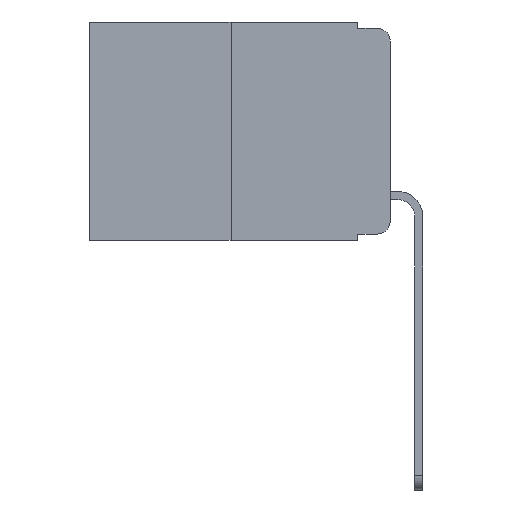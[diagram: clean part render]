
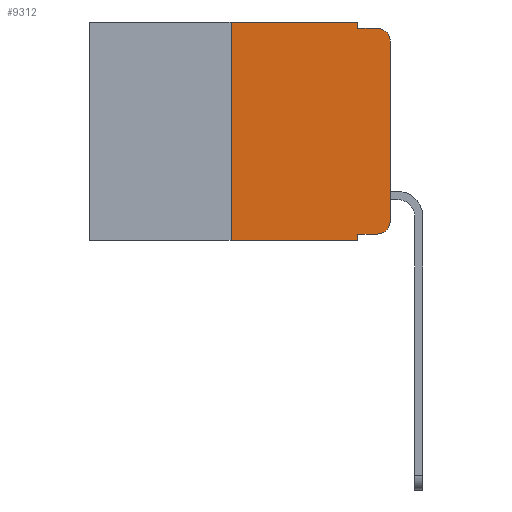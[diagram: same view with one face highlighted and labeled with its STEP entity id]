
A CAD part, left-side view. The second image highlights one B-rep face of the part: STEP entity #9312.
In plain terms, the highlighted planar face has unit normal (-1, 0, 0).
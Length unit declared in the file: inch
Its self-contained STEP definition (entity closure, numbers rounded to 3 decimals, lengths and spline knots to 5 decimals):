
#38 = EDGE_CURVE ( 'NONE', #4731, #8305, #4395, .T. ) ;
#246 = AXIS2_PLACEMENT_3D ( 'NONE', #2435, #3124, #7527 ) ;
#268 = VECTOR ( 'NONE', #2570, 39.37008 ) ;
#418 = DIRECTION ( 'NONE',  ( 0., 0., -1. ) ) ;
#618 = VERTEX_POINT ( 'NONE', #10409 ) ;
#759 = VERTEX_POINT ( 'NONE', #5820 ) ;
#871 = EDGE_CURVE ( 'NONE', #618, #2006, #10185, .T. ) ;
#977 = EDGE_CURVE ( 'NONE', #618, #759, #7016, .T. ) ;
#1231 = VERTEX_POINT ( 'NONE', #9079 ) ;
#1253 = LINE ( 'NONE', #7977, #6766 ) ;
#1435 = EDGE_LOOP ( 'NONE', ( #4017, #3977, #9161, #7987, #4756, #10477, #8982, #6982, #9890, #2852 ) ) ;
#1738 = LINE ( 'NONE', #4358, #268 ) ;
#1791 = VECTOR ( 'NONE', #7888, 39.37008 ) ;
#1796 = VERTEX_POINT ( 'NONE', #2466 ) ;
#1855 = CARTESIAN_POINT ( 'NONE',  ( 0., 0.051, 0. ) ) ;
#2006 = VERTEX_POINT ( 'NONE', #9600 ) ;
#2035 = EDGE_CURVE ( 'NONE', #1796, #4731, #2976, .T. ) ;
#2191 = CARTESIAN_POINT ( 'NONE',  ( 0., 0., 0. ) ) ;
#2269 = VERTEX_POINT ( 'NONE', #3836 ) ;
#2435 = CARTESIAN_POINT ( 'NONE',  ( 0., 0.02, -0.313 ) ) ;
#2466 = CARTESIAN_POINT ( 'NONE',  ( 0., 0., -0.313 ) ) ;
#2475 = DIRECTION ( 'NONE',  ( 0., 0., -1. ) ) ;
#2570 = DIRECTION ( 'NONE',  ( 0., -1., 0. ) ) ;
#2605 = FACE_OUTER_BOUND ( 'NONE', #1435, .T. ) ;
#2707 = VECTOR ( 'NONE', #9733, 39.37008 ) ;
#2758 = VECTOR ( 'NONE', #4250, 39.37008 ) ;
#2852 = ORIENTED_EDGE ( 'NONE', *, *, #8768, .T. ) ;
#2976 = LINE ( 'NONE', #2191, #7243 ) ;
#3007 = EDGE_CURVE ( 'NONE', #4421, #1231, #7748, .T. ) ;
#3092 = EDGE_CURVE ( 'NONE', #1231, #8305, #1738, .T. ) ;
#3124 = DIRECTION ( 'NONE',  ( -1., 0., 0. ) ) ;
#3449 = CARTESIAN_POINT ( 'NONE',  ( 0., 0.051, -0.333 ) ) ;
#3510 = CARTESIAN_POINT ( 'NONE',  ( 0., 0.051, 0. ) ) ;
#3558 = DIRECTION ( 'NONE',  ( 0., -1., 0. ) ) ;
#3601 = AXIS2_PLACEMENT_3D ( 'NONE', #4335, #9434, #2475 ) ;
#3698 = CARTESIAN_POINT ( 'NONE',  ( 0., 0.02, -0.01 ) ) ;
#3725 = CARTESIAN_POINT ( 'NONE',  ( 0., 0.473, -0.343 ) ) ;
#3809 = DIRECTION ( 'NONE',  ( 0., 0., 1. ) ) ;
#3836 = CARTESIAN_POINT ( 'NONE',  ( 0., 0.02, -0.333 ) ) ;
#3977 = ORIENTED_EDGE ( 'NONE', *, *, #38, .T. ) ;
#4017 = ORIENTED_EDGE ( 'NONE', *, *, #2035, .T. ) ;
#4250 = DIRECTION ( 'NONE',  ( 0., 0., -1. ) ) ;
#4335 = CARTESIAN_POINT ( 'NONE',  ( 0., 0.473, 0. ) ) ;
#4358 = CARTESIAN_POINT ( 'NONE',  ( 0., 0.051, -0.01 ) ) ;
#4395 = CIRCLE ( 'NONE', #10495, 0.02 ) ;
#4421 = VERTEX_POINT ( 'NONE', #1855 ) ;
#4731 = VERTEX_POINT ( 'NONE', #5989 ) ;
#4756 = ORIENTED_EDGE ( 'NONE', *, *, #9175, .F. ) ;
#4848 = VERTEX_POINT ( 'NONE', #6360 ) ;
#4989 = CARTESIAN_POINT ( 'NONE',  ( 0., 0.02, -0.03 ) ) ;
#5122 = CARTESIAN_POINT ( 'NONE',  ( 0., 0.25, 0. ) ) ;
#5555 = CIRCLE ( 'NONE', #246, 0.02 ) ;
#5820 = CARTESIAN_POINT ( 'NONE',  ( 0., 0.051, -0.343 ) ) ;
#5972 = DIRECTION ( 'NONE',  ( -1., 0., 0. ) ) ;
#5989 = CARTESIAN_POINT ( 'NONE',  ( 0., 0., -0.03 ) ) ;
#6360 = CARTESIAN_POINT ( 'NONE',  ( 0., 0.051, -0.333 ) ) ;
#6413 = LINE ( 'NONE', #7233, #2707 ) ;
#6766 = VECTOR ( 'NONE', #418, 39.37008 ) ;
#6982 = ORIENTED_EDGE ( 'NONE', *, *, #9575, .F. ) ;
#7016 = LINE ( 'NONE', #3725, #1791 ) ;
#7233 = CARTESIAN_POINT ( 'NONE',  ( 0., 0.473, 0. ) ) ;
#7243 = VECTOR ( 'NONE', #3809, 39.37008 ) ;
#7527 = DIRECTION ( 'NONE',  ( 0., 0., -1. ) ) ;
#7748 = LINE ( 'NONE', #3510, #2758 ) ;
#7888 = DIRECTION ( 'NONE',  ( 0., -1., 0. ) ) ;
#7977 = CARTESIAN_POINT ( 'NONE',  ( 0., 0.051, 0. ) ) ;
#7987 = ORIENTED_EDGE ( 'NONE', *, *, #3007, .F. ) ;
#8305 = VERTEX_POINT ( 'NONE', #3698 ) ;
#8440 = LINE ( 'NONE', #3449, #10113 ) ;
#8628 = VECTOR ( 'NONE', #9150, 39.37008 ) ;
#8768 = EDGE_CURVE ( 'NONE', #2269, #1796, #5555, .T. ) ;
#8982 = ORIENTED_EDGE ( 'NONE', *, *, #977, .T. ) ;
#9079 = CARTESIAN_POINT ( 'NONE',  ( 0., 0.051, -0.01 ) ) ;
#9150 = DIRECTION ( 'NONE',  ( 0., 0., 1. ) ) ;
#9161 = ORIENTED_EDGE ( 'NONE', *, *, #3092, .F. ) ;
#9175 = EDGE_CURVE ( 'NONE', #2006, #4421, #6413, .T. ) ;
#9312 = ADVANCED_FACE ( 'NONE', ( #2605 ), #10118, .F. ) ;
#9434 = DIRECTION ( 'NONE',  ( 1., 0., 0. ) ) ;
#9575 = EDGE_CURVE ( 'NONE', #4848, #759, #1253, .T. ) ;
#9600 = CARTESIAN_POINT ( 'NONE',  ( 0., 0.25, 0. ) ) ;
#9733 = DIRECTION ( 'NONE',  ( 0., -1., 0. ) ) ;
#9890 = ORIENTED_EDGE ( 'NONE', *, *, #10170, .T. ) ;
#10113 = VECTOR ( 'NONE', #3558, 39.37008 ) ;
#10118 = PLANE ( 'NONE',  #3601 ) ;
#10170 = EDGE_CURVE ( 'NONE', #4848, #2269, #8440, .T. ) ;
#10185 = LINE ( 'NONE', #5122, #8628 ) ;
#10409 = CARTESIAN_POINT ( 'NONE',  ( 0., 0.25, -0.343 ) ) ;
#10477 = ORIENTED_EDGE ( 'NONE', *, *, #871, .F. ) ;
#10495 = AXIS2_PLACEMENT_3D ( 'NONE', #4989, #5972, #10867 ) ;
#10867 = DIRECTION ( 'NONE',  ( 0., 0., -1. ) ) ;
